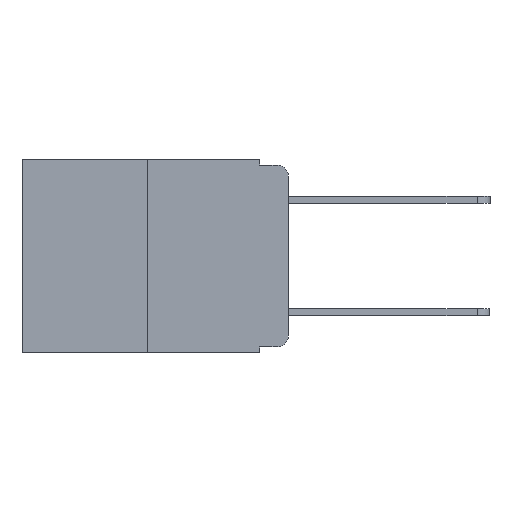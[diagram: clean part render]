
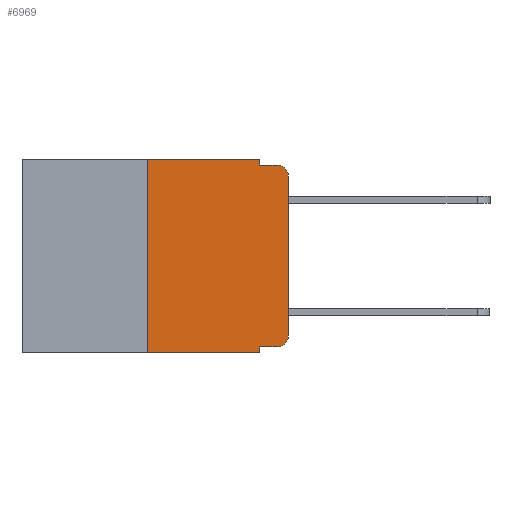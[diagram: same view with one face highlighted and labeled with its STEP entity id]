
A CAD part, left-side view. The second image highlights one B-rep face of the part: STEP entity #6969.
In plain terms, the highlighted planar face has unit normal (-1, 0, 0).
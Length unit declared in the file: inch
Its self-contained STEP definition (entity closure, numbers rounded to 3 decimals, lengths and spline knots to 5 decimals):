
#210 = VERTEX_POINT ( 'NONE', #15418 ) ;
#345 = PLANE ( 'NONE',  #15554 ) ;
#450 = VERTEX_POINT ( 'NONE', #5765 ) ;
#525 = VECTOR ( 'NONE', #2213, 39.37008 ) ;
#662 = LINE ( 'NONE', #13954, #10134 ) ;
#761 = DIRECTION ( 'NONE',  ( 0., 0., -1. ) ) ;
#998 = LINE ( 'NONE', #9775, #14324 ) ;
#1045 = DIRECTION ( 'NONE',  ( 0., -1., 0. ) ) ;
#1185 = ORIENTED_EDGE ( 'NONE', *, *, #8969, .T. ) ;
#1836 = CARTESIAN_POINT ( 'NONE',  ( 0., 0.473, -0.343 ) ) ;
#2213 = DIRECTION ( 'NONE',  ( 0., 0., 1. ) ) ;
#2238 = DIRECTION ( 'NONE',  ( 0., 0., 1. ) ) ;
#2360 = CARTESIAN_POINT ( 'NONE',  ( 0., 0.02, -0.03 ) ) ;
#2397 = DIRECTION ( 'NONE',  ( 0., 0., -1. ) ) ;
#2791 = VERTEX_POINT ( 'NONE', #14654 ) ;
#2812 = LINE ( 'NONE', #1836, #9509 ) ;
#3167 = CIRCLE ( 'NONE', #11927, 0.02 ) ;
#3475 = DIRECTION ( 'NONE',  ( 0., 0., -1. ) ) ;
#3634 = DIRECTION ( 'NONE',  ( 0., 0., -1. ) ) ;
#3787 = DIRECTION ( 'NONE',  ( -1., 0., 0. ) ) ;
#4747 = VERTEX_POINT ( 'NONE', #14909 ) ;
#4988 = ORIENTED_EDGE ( 'NONE', *, *, #8862, .F. ) ;
#5765 = CARTESIAN_POINT ( 'NONE',  ( 0., 0.25, -0.343 ) ) ;
#5786 = ORIENTED_EDGE ( 'NONE', *, *, #8394, .T. ) ;
#5830 = VECTOR ( 'NONE', #7398, 39.37008 ) ;
#6122 = CARTESIAN_POINT ( 'NONE',  ( 0., 0.051, -0.333 ) ) ;
#6347 = ORIENTED_EDGE ( 'NONE', *, *, #8810, .T. ) ;
#6607 = ORIENTED_EDGE ( 'NONE', *, *, #8952, .T. ) ;
#6609 = LINE ( 'NONE', #9937, #12869 ) ;
#6675 = EDGE_CURVE ( 'NONE', #4747, #14165, #662, .T. ) ;
#6798 = CARTESIAN_POINT ( 'NONE',  ( 0., 0.02, -0.01 ) ) ;
#6818 = CARTESIAN_POINT ( 'NONE',  ( 0., 0.02, -0.333 ) ) ;
#6969 = ADVANCED_FACE ( 'NONE', ( #12790 ), #345, .F. ) ;
#7398 = DIRECTION ( 'NONE',  ( 0., -1., 0. ) ) ;
#7419 = CARTESIAN_POINT ( 'NONE',  ( 0., 0.051, -0.01 ) ) ;
#7766 = CARTESIAN_POINT ( 'NONE',  ( 0., 0.051, -0.343 ) ) ;
#7819 = VERTEX_POINT ( 'NONE', #10259 ) ;
#8077 = VERTEX_POINT ( 'NONE', #7766 ) ;
#8238 = LINE ( 'NONE', #10970, #525 ) ;
#8394 = EDGE_CURVE ( 'NONE', #450, #8077, #2812, .T. ) ;
#8597 = VERTEX_POINT ( 'NONE', #14967 ) ;
#8627 = LINE ( 'NONE', #7419, #9479 ) ;
#8808 = EDGE_CURVE ( 'NONE', #8597, #7819, #16114, .T. ) ;
#8810 = EDGE_CURVE ( 'NONE', #7819, #10817, #3167, .T. ) ;
#8847 = CIRCLE ( 'NONE', #14838, 0.02 ) ;
#8862 = EDGE_CURVE ( 'NONE', #210, #10817, #8627, .T. ) ;
#8911 = EDGE_CURVE ( 'NONE', #14165, #210, #998, .T. ) ;
#8915 = EDGE_CURVE ( 'NONE', #450, #4747, #8238, .T. ) ;
#8946 = EDGE_CURVE ( 'NONE', #2791, #8077, #6609, .T. ) ;
#8952 = EDGE_CURVE ( 'NONE', #2791, #13684, #15586, .T. ) ;
#8969 = EDGE_CURVE ( 'NONE', #13684, #8597, #8847, .T. ) ;
#9479 = VECTOR ( 'NONE', #1045, 39.37008 ) ;
#9509 = VECTOR ( 'NONE', #10650, 39.37008 ) ;
#9775 = CARTESIAN_POINT ( 'NONE',  ( 0., 0.051, 0. ) ) ;
#9853 = CARTESIAN_POINT ( 'NONE',  ( 0., 0., 0. ) ) ;
#9937 = CARTESIAN_POINT ( 'NONE',  ( 0., 0.051, 0. ) ) ;
#9979 = ORIENTED_EDGE ( 'NONE', *, *, #8915, .F. ) ;
#10125 = ORIENTED_EDGE ( 'NONE', *, *, #8911, .F. ) ;
#10134 = VECTOR ( 'NONE', #15623, 39.37008 ) ;
#10152 = ORIENTED_EDGE ( 'NONE', *, *, #6675, .F. ) ;
#10259 = CARTESIAN_POINT ( 'NONE',  ( 0., 0., -0.03 ) ) ;
#10280 = EDGE_LOOP ( 'NONE', ( #14614, #6347, #4988, #10125, #10152, #9979, #5786, #14653, #6607, #1185 ) ) ;
#10650 = DIRECTION ( 'NONE',  ( 0., -1., 0. ) ) ;
#10817 = VERTEX_POINT ( 'NONE', #6798 ) ;
#10918 = DIRECTION ( 'NONE',  ( 1., 0., 0. ) ) ;
#10970 = CARTESIAN_POINT ( 'NONE',  ( 0., 0.25, 0. ) ) ;
#11080 = DIRECTION ( 'NONE',  ( -1., 0., 0. ) ) ;
#11089 = CARTESIAN_POINT ( 'NONE',  ( 0., 0.051, 0. ) ) ;
#11230 = CARTESIAN_POINT ( 'NONE',  ( 0., 0.02, -0.313 ) ) ;
#11927 = AXIS2_PLACEMENT_3D ( 'NONE', #2360, #11080, #3634 ) ;
#12482 = DIRECTION ( 'NONE',  ( 0., 0., -1. ) ) ;
#12683 = VECTOR ( 'NONE', #2238, 39.37008 ) ;
#12790 = FACE_OUTER_BOUND ( 'NONE', #10280, .T. ) ;
#12815 = CARTESIAN_POINT ( 'NONE',  ( 0., 0.473, 0. ) ) ;
#12869 = VECTOR ( 'NONE', #2397, 39.37008 ) ;
#13684 = VERTEX_POINT ( 'NONE', #6818 ) ;
#13954 = CARTESIAN_POINT ( 'NONE',  ( 0., 0.473, 0. ) ) ;
#14165 = VERTEX_POINT ( 'NONE', #11089 ) ;
#14324 = VECTOR ( 'NONE', #761, 39.37008 ) ;
#14614 = ORIENTED_EDGE ( 'NONE', *, *, #8808, .T. ) ;
#14653 = ORIENTED_EDGE ( 'NONE', *, *, #8946, .F. ) ;
#14654 = CARTESIAN_POINT ( 'NONE',  ( 0., 0.051, -0.333 ) ) ;
#14838 = AXIS2_PLACEMENT_3D ( 'NONE', #11230, #3787, #12482 ) ;
#14909 = CARTESIAN_POINT ( 'NONE',  ( 0., 0.25, 0. ) ) ;
#14967 = CARTESIAN_POINT ( 'NONE',  ( 0., 0., -0.313 ) ) ;
#15418 = CARTESIAN_POINT ( 'NONE',  ( 0., 0.051, -0.01 ) ) ;
#15554 = AXIS2_PLACEMENT_3D ( 'NONE', #12815, #10918, #3475 ) ;
#15586 = LINE ( 'NONE', #6122, #5830 ) ;
#15623 = DIRECTION ( 'NONE',  ( 0., -1., 0. ) ) ;
#16114 = LINE ( 'NONE', #9853, #12683 ) ;
